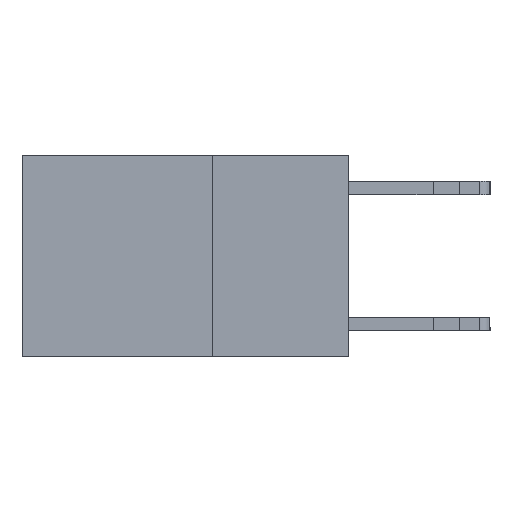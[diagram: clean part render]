
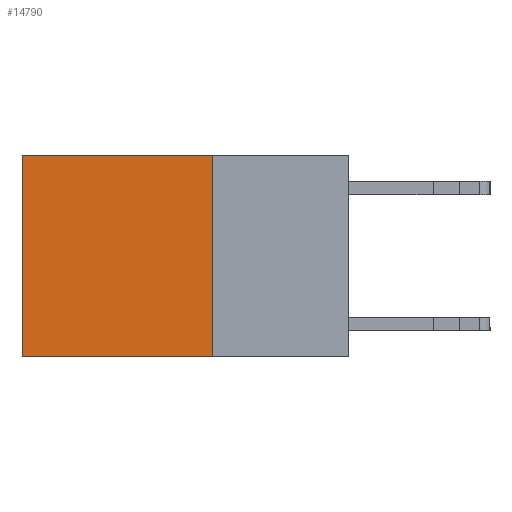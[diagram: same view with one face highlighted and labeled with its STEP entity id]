
A CAD part, left-side view. The second image highlights one B-rep face of the part: STEP entity #14790.
In plain terms, the highlighted planar face has unit normal (-1, 0, 0).
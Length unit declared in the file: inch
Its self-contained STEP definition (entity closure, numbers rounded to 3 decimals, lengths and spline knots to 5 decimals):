
#296 = EDGE_CURVE ( 'NONE', #16238, #18038, #1120, .T. ) ;
#1120 = LINE ( 'NONE', #15778, #4087 ) ;
#1831 = EDGE_CURVE ( 'NONE', #18038, #12183, #2117, .T. ) ;
#2117 = LINE ( 'NONE', #13044, #15090 ) ;
#2988 = EDGE_CURVE ( 'NONE', #16238, #18411, #5444, .T. ) ;
#3230 = AXIS2_PLACEMENT_3D ( 'NONE', #16088, #4033, #24436 ) ;
#3878 = CARTESIAN_POINT ( 'NONE',  ( 0.2625, 0.6, -0.37 ) ) ;
#4033 = DIRECTION ( 'NONE',  ( 1., 0., 0. ) ) ;
#4087 = VECTOR ( 'NONE', #24115, 39.37008 ) ;
#5444 = LINE ( 'NONE', #26344, #16439 ) ;
#7084 = ORIENTED_EDGE ( 'NONE', *, *, #11831, .F. ) ;
#7490 = ORIENTED_EDGE ( 'NONE', *, *, #2988, .F. ) ;
#8389 = ORIENTED_EDGE ( 'NONE', *, *, #296, .T. ) ;
#10602 = DIRECTION ( 'NONE',  ( 0., 0., -1. ) ) ;
#11010 = CARTESIAN_POINT ( 'NONE',  ( 0.2625, 0.25, 0. ) ) ;
#11831 = EDGE_CURVE ( 'NONE', #18411, #12183, #22787, .T. ) ;
#12183 = VERTEX_POINT ( 'NONE', #3878 ) ;
#12381 = CARTESIAN_POINT ( 'NONE',  ( 0.2625, 0.25, -0.37 ) ) ;
#13044 = CARTESIAN_POINT ( 'NONE',  ( 0.2625, 0.6, 0. ) ) ;
#13786 = DIRECTION ( 'NONE',  ( 0., 0., -1. ) ) ;
#14790 = ADVANCED_FACE ( 'NONE', ( #24297 ), #15950, .F. ) ;
#15090 = VECTOR ( 'NONE', #10602, 39.37008 ) ;
#15778 = CARTESIAN_POINT ( 'NONE',  ( 0.2625, 0.25, 0. ) ) ;
#15950 = PLANE ( 'NONE',  #3230 ) ;
#16088 = CARTESIAN_POINT ( 'NONE',  ( 0.2625, 0.25, 0. ) ) ;
#16238 = VERTEX_POINT ( 'NONE', #11010 ) ;
#16439 = VECTOR ( 'NONE', #13786, 39.37008 ) ;
#16636 = DIRECTION ( 'NONE',  ( 0., 1., 0. ) ) ;
#17965 = EDGE_LOOP ( 'NONE', ( #22385, #7084, #7490, #8389 ) ) ;
#18038 = VERTEX_POINT ( 'NONE', #25211 ) ;
#18411 = VERTEX_POINT ( 'NONE', #22327 ) ;
#22327 = CARTESIAN_POINT ( 'NONE',  ( 0.2625, 0.25, -0.37 ) ) ;
#22385 = ORIENTED_EDGE ( 'NONE', *, *, #1831, .T. ) ;
#22787 = LINE ( 'NONE', #12381, #23400 ) ;
#23400 = VECTOR ( 'NONE', #16636, 39.37008 ) ;
#24115 = DIRECTION ( 'NONE',  ( 0., 1., 0. ) ) ;
#24297 = FACE_OUTER_BOUND ( 'NONE', #17965, .T. ) ;
#24436 = DIRECTION ( 'NONE',  ( 0., 0., -1. ) ) ;
#25211 = CARTESIAN_POINT ( 'NONE',  ( 0.2625, 0.6, 0. ) ) ;
#26344 = CARTESIAN_POINT ( 'NONE',  ( 0.2625, 0.25, 0. ) ) ;
